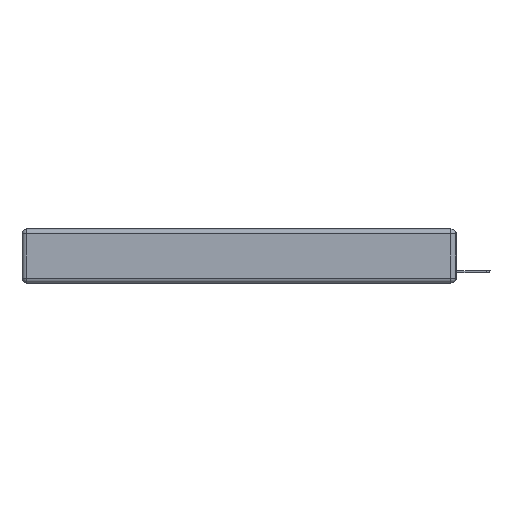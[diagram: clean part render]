
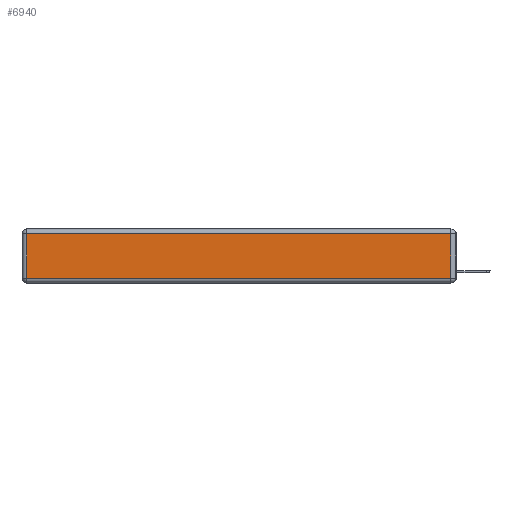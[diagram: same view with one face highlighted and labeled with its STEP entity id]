
A CAD part, left-side view. The second image highlights one B-rep face of the part: STEP entity #6940.
In plain terms, the highlighted planar face has unit normal (-1, 0, 0).
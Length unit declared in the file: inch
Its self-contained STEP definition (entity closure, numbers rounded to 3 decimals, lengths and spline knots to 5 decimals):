
#287 = CARTESIAN_POINT ( 'NONE',  ( 0., 0.03, -0.343 ) ) ;
#612 = AXIS2_PLACEMENT_3D ( 'NONE', #13705, #13789, #5764 ) ;
#957 = EDGE_CURVE ( 'NONE', #9930, #3205, #2397, .T. ) ;
#1123 = CARTESIAN_POINT ( 'NONE',  ( 0., 2.72, -0.03 ) ) ;
#1418 = ORIENTED_EDGE ( 'NONE', *, *, #10065, .T. ) ;
#1535 = CARTESIAN_POINT ( 'NONE',  ( 0., 0.03, -0.03 ) ) ;
#2092 = ORIENTED_EDGE ( 'NONE', *, *, #957, .T. ) ;
#2397 = LINE ( 'NONE', #15815, #2931 ) ;
#2931 = VECTOR ( 'NONE', #9372, 39.37008 ) ;
#3069 = EDGE_LOOP ( 'NONE', ( #8159, #1418, #2092, #13917 ) ) ;
#3107 = FACE_OUTER_BOUND ( 'NONE', #3069, .T. ) ;
#3205 = VERTEX_POINT ( 'NONE', #1123 ) ;
#4214 = CARTESIAN_POINT ( 'NONE',  ( 0., 2.72, -0.343 ) ) ;
#4380 = DIRECTION ( 'NONE',  ( 0., 0., -1. ) ) ;
#4711 = PLANE ( 'NONE',  #612 ) ;
#5764 = DIRECTION ( 'NONE',  ( 0., 0., 1. ) ) ;
#6671 = VERTEX_POINT ( 'NONE', #8894 ) ;
#6923 = CARTESIAN_POINT ( 'NONE',  ( 0., 2.72, -0.313 ) ) ;
#6940 = ADVANCED_FACE ( 'NONE', ( #3107 ), #4711, .T. ) ;
#7144 = VECTOR ( 'NONE', #15203, 39.37008 ) ;
#8159 = ORIENTED_EDGE ( 'NONE', *, *, #15857, .T. ) ;
#8608 = VERTEX_POINT ( 'NONE', #6923 ) ;
#8894 = CARTESIAN_POINT ( 'NONE',  ( 0., 0.03, -0.313 ) ) ;
#9137 = DIRECTION ( 'NONE',  ( 0., -1., 0. ) ) ;
#9372 = DIRECTION ( 'NONE',  ( 0., 1., 0. ) ) ;
#9586 = VECTOR ( 'NONE', #9137, 39.37008 ) ;
#9930 = VERTEX_POINT ( 'NONE', #1535 ) ;
#10065 = EDGE_CURVE ( 'NONE', #6671, #9930, #12386, .T. ) ;
#11173 = LINE ( 'NONE', #4214, #16098 ) ;
#12386 = LINE ( 'NONE', #287, #7144 ) ;
#13705 = CARTESIAN_POINT ( 'NONE',  ( 0., 0., -0.343 ) ) ;
#13789 = DIRECTION ( 'NONE',  ( -1., 0., 0. ) ) ;
#13917 = ORIENTED_EDGE ( 'NONE', *, *, #16865, .T. ) ;
#15203 = DIRECTION ( 'NONE',  ( 0., 0., 1. ) ) ;
#15815 = CARTESIAN_POINT ( 'NONE',  ( 0., 2.75, -0.03 ) ) ;
#15857 = EDGE_CURVE ( 'NONE', #8608, #6671, #16027, .T. ) ;
#16027 = LINE ( 'NONE', #17089, #9586 ) ;
#16098 = VECTOR ( 'NONE', #4380, 39.37008 ) ;
#16865 = EDGE_CURVE ( 'NONE', #3205, #8608, #11173, .T. ) ;
#17089 = CARTESIAN_POINT ( 'NONE',  ( 0., 0., -0.313 ) ) ;
